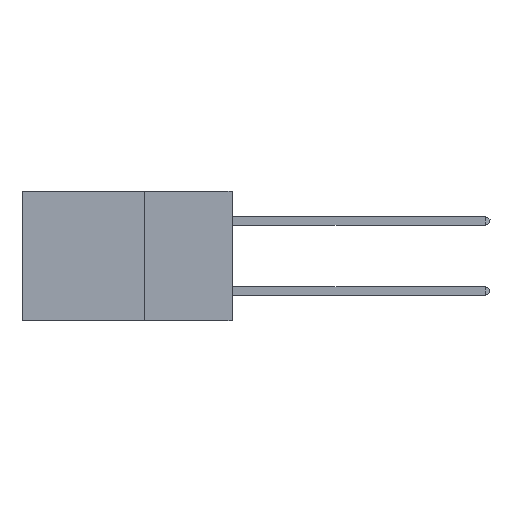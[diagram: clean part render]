
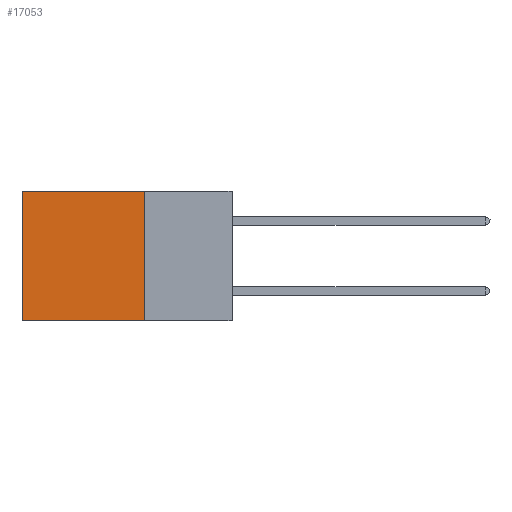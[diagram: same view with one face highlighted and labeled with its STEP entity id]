
A CAD part, left-side view. The second image highlights one B-rep face of the part: STEP entity #17053.
In plain terms, the highlighted planar face has unit normal (-1, 0, 0).
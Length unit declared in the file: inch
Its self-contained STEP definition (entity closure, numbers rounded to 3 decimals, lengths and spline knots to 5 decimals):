
#1020 = ORIENTED_EDGE ( 'NONE', *, *, #18737, .F. ) ;
#1304 = ORIENTED_EDGE ( 'NONE', *, *, #20689, .T. ) ;
#2300 = LINE ( 'NONE', #3565, #23397 ) ;
#2431 = PLANE ( 'NONE',  #7707 ) ;
#2615 = ORIENTED_EDGE ( 'NONE', *, *, #23769, .F. ) ;
#2812 = FACE_OUTER_BOUND ( 'NONE', #19147, .T. ) ;
#3351 = VECTOR ( 'NONE', #8581, 39.37008 ) ;
#3565 = CARTESIAN_POINT ( 'NONE',  ( 0.2875, 0.25, 0. ) ) ;
#5742 = VECTOR ( 'NONE', #25082, 39.37008 ) ;
#6181 = DIRECTION ( 'NONE',  ( 0., 0., -1. ) ) ;
#7666 = EDGE_CURVE ( 'NONE', #26686, #26354, #2300, .T. ) ;
#7707 = AXIS2_PLACEMENT_3D ( 'NONE', #26262, #21935, #17575 ) ;
#8207 = VECTOR ( 'NONE', #6181, 39.37008 ) ;
#8581 = DIRECTION ( 'NONE',  ( 0., 1., 0. ) ) ;
#9164 = ORIENTED_EDGE ( 'NONE', *, *, #7666, .T. ) ;
#9693 = CARTESIAN_POINT ( 'NONE',  ( 0.2875, 0.25, 0. ) ) ;
#13759 = VERTEX_POINT ( 'NONE', #26680 ) ;
#14026 = LINE ( 'NONE', #16893, #8207 ) ;
#14849 = VERTEX_POINT ( 'NONE', #19604 ) ;
#16893 = CARTESIAN_POINT ( 'NONE',  ( 0.2875, 0.6, 0. ) ) ;
#17053 = ADVANCED_FACE ( 'NONE', ( #2812 ), #2431, .F. ) ;
#17575 = DIRECTION ( 'NONE',  ( 0., 0., -1. ) ) ;
#17804 = CARTESIAN_POINT ( 'NONE',  ( 0.2875, 0.6, 0. ) ) ;
#18737 = EDGE_CURVE ( 'NONE', #26686, #13759, #19352, .T. ) ;
#19147 = EDGE_LOOP ( 'NONE', ( #1304, #2615, #1020, #9164 ) ) ;
#19352 = LINE ( 'NONE', #22913, #5742 ) ;
#19604 = CARTESIAN_POINT ( 'NONE',  ( 0.2875, 0.6, -0.37 ) ) ;
#20689 = EDGE_CURVE ( 'NONE', #26354, #14849, #14026, .T. ) ;
#21148 = DIRECTION ( 'NONE',  ( 0., 1., 0. ) ) ;
#21725 = CARTESIAN_POINT ( 'NONE',  ( 0.2875, 0.25, -0.37 ) ) ;
#21935 = DIRECTION ( 'NONE',  ( 1., 0., 0. ) ) ;
#22913 = CARTESIAN_POINT ( 'NONE',  ( 0.2875, 0.25, 0. ) ) ;
#23397 = VECTOR ( 'NONE', #21148, 39.37008 ) ;
#23769 = EDGE_CURVE ( 'NONE', #13759, #14849, #24767, .T. ) ;
#24767 = LINE ( 'NONE', #21725, #3351 ) ;
#25082 = DIRECTION ( 'NONE',  ( 0., 0., -1. ) ) ;
#26262 = CARTESIAN_POINT ( 'NONE',  ( 0.2875, 0.25, 0. ) ) ;
#26354 = VERTEX_POINT ( 'NONE', #17804 ) ;
#26680 = CARTESIAN_POINT ( 'NONE',  ( 0.2875, 0.25, -0.37 ) ) ;
#26686 = VERTEX_POINT ( 'NONE', #9693 ) ;
